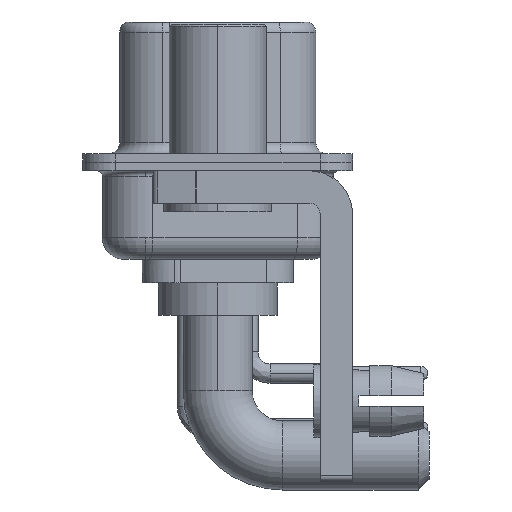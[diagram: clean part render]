
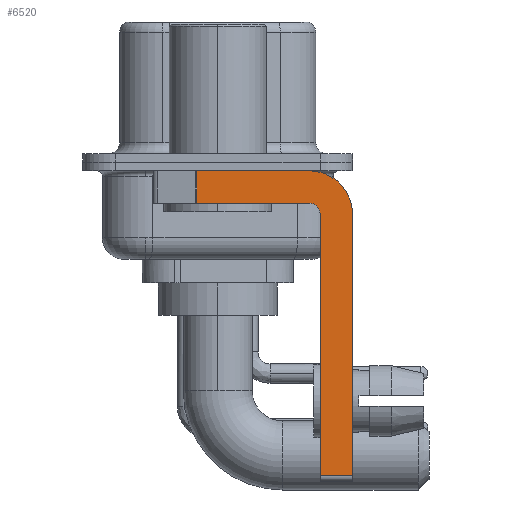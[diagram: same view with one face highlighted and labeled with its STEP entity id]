
A CAD part, left-side view. The second image highlights one B-rep face of the part: STEP entity #6520.
In plain terms, the highlighted planar face has unit normal (-1, 0, 0).
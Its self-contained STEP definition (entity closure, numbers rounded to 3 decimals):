
#190 = ORIENTED_EDGE ( 'NONE', *, *, #12456, .T. ) ;
#218 = CARTESIAN_POINT ( 'NONE',  ( -2.9, -4.25, -2.4 ) ) ;
#471 = DIRECTION ( 'NONE',  ( 0., 0., -1. ) ) ;
#711 = DIRECTION ( 'NONE',  ( -1., 0., 0. ) ) ;
#837 = AXIS2_PLACEMENT_3D ( 'NONE', #218, #4175, #471 ) ;
#1198 = CARTESIAN_POINT ( 'NONE',  ( -2.9, 3., -0.4 ) ) ;
#1219 = CARTESIAN_POINT ( 'NONE',  ( -2.9, -6.25, -14.55 ) ) ;
#1950 = EDGE_LOOP ( 'NONE', ( #2295, #11306, #2559, #6446, #12051, #190, #8021, #12296 ) ) ;
#2082 = CARTESIAN_POINT ( 'NONE',  ( -2.9, -4.25, -0.4 ) ) ;
#2295 = ORIENTED_EDGE ( 'NONE', *, *, #12534, .F. ) ;
#2344 = PLANE ( 'NONE',  #11786 ) ;
#2552 = EDGE_CURVE ( 'NONE', #22353, #13977, #14392, .T. ) ;
#2559 = ORIENTED_EDGE ( 'NONE', *, *, #2552, .F. ) ;
#2816 = LINE ( 'NONE', #1198, #16629 ) ;
#4175 = DIRECTION ( 'NONE',  ( 1., 0., 0. ) ) ;
#4198 = EDGE_CURVE ( 'NONE', #20788, #8579, #8124, .T. ) ;
#4646 = CARTESIAN_POINT ( 'NONE',  ( -2.9, 0.978, -1.9 ) ) ;
#4777 = VECTOR ( 'NONE', #22049, 1000. ) ;
#5722 = EDGE_CURVE ( 'NONE', #14292, #19433, #23936, .T. ) ;
#5938 = VECTOR ( 'NONE', #11960, 1000. ) ;
#6414 = DIRECTION ( 'NONE',  ( 0., 0., -1. ) ) ;
#6446 = ORIENTED_EDGE ( 'NONE', *, *, #13648, .F. ) ;
#6520 = ADVANCED_FACE ( 'NONE', ( #19543 ), #2344, .F. ) ;
#7102 = CARTESIAN_POINT ( 'NONE',  ( -2.9, -4.75, -2.4 ) ) ;
#8021 = ORIENTED_EDGE ( 'NONE', *, *, #5722, .F. ) ;
#8124 = LINE ( 'NONE', #10104, #14580 ) ;
#8145 = DIRECTION ( 'NONE',  ( 1., 0., 0. ) ) ;
#8199 = EDGE_CURVE ( 'NONE', #8349, #14292, #11487, .T. ) ;
#8209 = CARTESIAN_POINT ( 'NONE',  ( -2.9, -6.25, -2.4 ) ) ;
#8349 = VERTEX_POINT ( 'NONE', #2082 ) ;
#8579 = VERTEX_POINT ( 'NONE', #7102 ) ;
#8810 = VECTOR ( 'NONE', #23049, 1000. ) ;
#9740 = DIRECTION ( 'NONE',  ( 0., 0., 1. ) ) ;
#10104 = CARTESIAN_POINT ( 'NONE',  ( -2.9, -4.75, -14.8 ) ) ;
#11138 = VECTOR ( 'NONE', #19737, 1000. ) ;
#11306 = ORIENTED_EDGE ( 'NONE', *, *, #19762, .T. ) ;
#11487 = CIRCLE ( 'NONE', #837, 2. ) ;
#11786 = AXIS2_PLACEMENT_3D ( 'NONE', #15460, #8145, #6414 ) ;
#11830 = LINE ( 'NONE', #20872, #5938 ) ;
#11960 = DIRECTION ( 'NONE',  ( 0., -1., 0. ) ) ;
#12051 = ORIENTED_EDGE ( 'NONE', *, *, #4198, .F. ) ;
#12296 = ORIENTED_EDGE ( 'NONE', *, *, #8199, .F. ) ;
#12456 = EDGE_CURVE ( 'NONE', #20788, #19433, #11830, .T. ) ;
#12534 = EDGE_CURVE ( 'NONE', #23051, #8349, #2816, .T. ) ;
#13648 = EDGE_CURVE ( 'NONE', #8579, #22353, #19406, .T. ) ;
#13733 = CARTESIAN_POINT ( 'NONE',  ( -2.9, -4.25, -1.9 ) ) ;
#13977 = VERTEX_POINT ( 'NONE', #15034 ) ;
#14080 = CARTESIAN_POINT ( 'NONE',  ( -2.9, 0.978, -0.4 ) ) ;
#14292 = VERTEX_POINT ( 'NONE', #8209 ) ;
#14392 = LINE ( 'NONE', #15113, #8810 ) ;
#14503 = CARTESIAN_POINT ( 'NONE',  ( -2.9, -6.25, -2.4 ) ) ;
#14580 = VECTOR ( 'NONE', #15928, 1000. ) ;
#15034 = CARTESIAN_POINT ( 'NONE',  ( -2.9, 0.978, -1.9 ) ) ;
#15113 = CARTESIAN_POINT ( 'NONE',  ( -2.9, -4.25, -1.9 ) ) ;
#15460 = CARTESIAN_POINT ( 'NONE',  ( -2.9, -4.25, -2.4 ) ) ;
#15928 = DIRECTION ( 'NONE',  ( 0., 0., 1. ) ) ;
#16629 = VECTOR ( 'NONE', #19996, 1000. ) ;
#17758 = LINE ( 'NONE', #4646, #11138 ) ;
#18006 = CARTESIAN_POINT ( 'NONE',  ( -2.9, -4.75, -14.55 ) ) ;
#18221 = AXIS2_PLACEMENT_3D ( 'NONE', #19527, #711, #9740 ) ;
#19406 = CIRCLE ( 'NONE', #18221, 0.5 ) ;
#19433 = VERTEX_POINT ( 'NONE', #1219 ) ;
#19527 = CARTESIAN_POINT ( 'NONE',  ( -2.9, -4.25, -2.4 ) ) ;
#19543 = FACE_OUTER_BOUND ( 'NONE', #1950, .T. ) ;
#19737 = DIRECTION ( 'NONE',  ( 0., 0., -1. ) ) ;
#19762 = EDGE_CURVE ( 'NONE', #23051, #13977, #17758, .T. ) ;
#19996 = DIRECTION ( 'NONE',  ( 0., -1., 0. ) ) ;
#20788 = VERTEX_POINT ( 'NONE', #18006 ) ;
#20872 = CARTESIAN_POINT ( 'NONE',  ( -2.9, -4.25, -14.55 ) ) ;
#22049 = DIRECTION ( 'NONE',  ( 0., 0., -1. ) ) ;
#22353 = VERTEX_POINT ( 'NONE', #13733 ) ;
#23049 = DIRECTION ( 'NONE',  ( 0., 1., 0. ) ) ;
#23051 = VERTEX_POINT ( 'NONE', #14080 ) ;
#23936 = LINE ( 'NONE', #14503, #4777 ) ;
